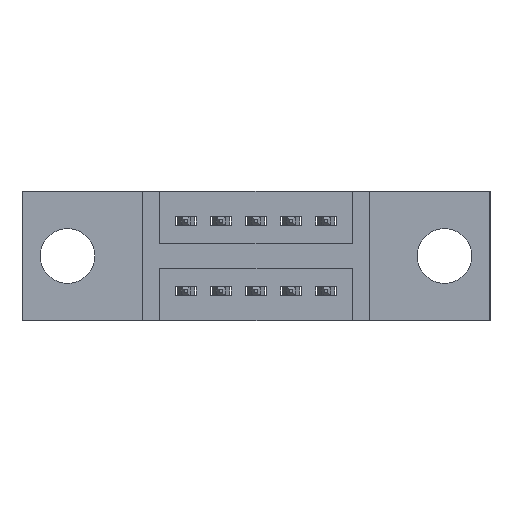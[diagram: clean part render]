
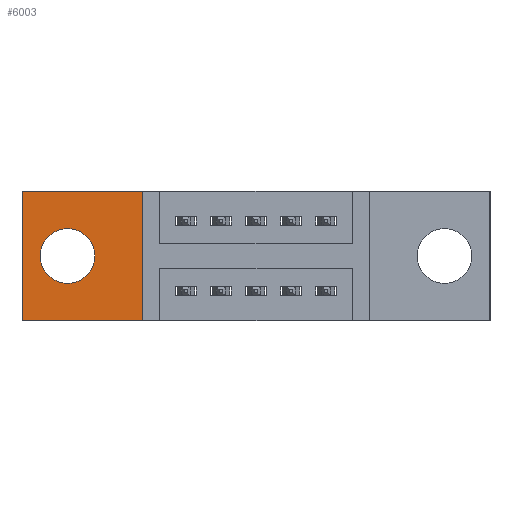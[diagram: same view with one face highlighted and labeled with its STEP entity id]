
A CAD part, front view. The second image highlights one B-rep face of the part: STEP entity #6003.
In plain terms, the highlighted planar face has unit normal (0, -1, 0).
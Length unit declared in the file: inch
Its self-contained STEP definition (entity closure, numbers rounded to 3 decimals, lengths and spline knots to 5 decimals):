
#191 = CIRCLE ( 'NONE', #6354, 0.078 ) ;
#339 = VERTEX_POINT ( 'NONE', #7462 ) ;
#435 = ORIENTED_EDGE ( 'NONE', *, *, #7340, .F. ) ;
#459 = ORIENTED_EDGE ( 'NONE', *, *, #895, .T. ) ;
#604 = CARTESIAN_POINT ( 'NONE',  ( 0.3425, 0.17, 0. ) ) ;
#630 = DIRECTION ( 'NONE',  ( 0., 0., 1. ) ) ;
#660 = DIRECTION ( 'NONE',  ( 1., 0., 0. ) ) ;
#766 = VERTEX_POINT ( 'NONE', #769 ) ;
#769 = CARTESIAN_POINT ( 'NONE',  ( 0.13, 0.17, -0.263 ) ) ;
#827 = ORIENTED_EDGE ( 'NONE', *, *, #8716, .F. ) ;
#895 = EDGE_CURVE ( 'NONE', #339, #7707, #3642, .T. ) ;
#1202 = CARTESIAN_POINT ( 'NONE',  ( 0., 0.17, -0.37 ) ) ;
#1680 = DIRECTION ( 'NONE',  ( 0., 0., -1. ) ) ;
#2078 = VERTEX_POINT ( 'NONE', #5749 ) ;
#2148 = EDGE_CURVE ( 'NONE', #7707, #3746, #3924, .T. ) ;
#2295 = ORIENTED_EDGE ( 'NONE', *, *, #2148, .T. ) ;
#2442 = VECTOR ( 'NONE', #2917, 39.37008 ) ;
#2473 = EDGE_CURVE ( 'NONE', #3746, #4569, #2979, .T. ) ;
#2695 = AXIS2_PLACEMENT_3D ( 'NONE', #4217, #8788, #4899 ) ;
#2917 = DIRECTION ( 'NONE',  ( 0., 0., -1. ) ) ;
#2979 = LINE ( 'NONE', #7596, #4770 ) ;
#3642 = LINE ( 'NONE', #1202, #6885 ) ;
#3746 = VERTEX_POINT ( 'NONE', #5152 ) ;
#3902 = CARTESIAN_POINT ( 'NONE',  ( 0.13, 0.17, -0.185 ) ) ;
#3924 = LINE ( 'NONE', #604, #7162 ) ;
#4132 = FACE_OUTER_BOUND ( 'NONE', #7929, .T. ) ;
#4217 = CARTESIAN_POINT ( 'NONE',  ( 0.13, 0.17, -0.185 ) ) ;
#4569 = VERTEX_POINT ( 'NONE', #7557 ) ;
#4583 = DIRECTION ( 'NONE',  ( 0., 0., -1. ) ) ;
#4770 = VECTOR ( 'NONE', #7552, 39.37008 ) ;
#4899 = DIRECTION ( 'NONE',  ( 0., 0., -1. ) ) ;
#4927 = ORIENTED_EDGE ( 'NONE', *, *, #8807, .T. ) ;
#4945 = CIRCLE ( 'NONE', #2695, 0.078 ) ;
#5152 = CARTESIAN_POINT ( 'NONE',  ( 0.3425, 0.17, 0. ) ) ;
#5584 = CARTESIAN_POINT ( 'NONE',  ( 0.3425, 0.17, -0.37 ) ) ;
#5749 = CARTESIAN_POINT ( 'NONE',  ( 0.13, 0.17, -0.107 ) ) ;
#5813 = DIRECTION ( 'NONE',  ( 0., -1., 0. ) ) ;
#5856 = FACE_BOUND ( 'NONE', #6951, .T. ) ;
#6003 = ADVANCED_FACE ( 'NONE', ( #5856, #4132 ), #7057, .T. ) ;
#6025 = LINE ( 'NONE', #8849, #2442 ) ;
#6354 = AXIS2_PLACEMENT_3D ( 'NONE', #3902, #8492, #4583 ) ;
#6885 = VECTOR ( 'NONE', #660, 39.37008 ) ;
#6951 = EDGE_LOOP ( 'NONE', ( #435, #827 ) ) ;
#7057 = PLANE ( 'NONE',  #7858 ) ;
#7162 = VECTOR ( 'NONE', #630, 39.37008 ) ;
#7340 = EDGE_CURVE ( 'NONE', #2078, #766, #191, .T. ) ;
#7462 = CARTESIAN_POINT ( 'NONE',  ( 0., 0.17, -0.37 ) ) ;
#7552 = DIRECTION ( 'NONE',  ( -1., 0., 0. ) ) ;
#7557 = CARTESIAN_POINT ( 'NONE',  ( 0., 0.17, 0. ) ) ;
#7596 = CARTESIAN_POINT ( 'NONE',  ( 0., 0.17, 0. ) ) ;
#7707 = VERTEX_POINT ( 'NONE', #5584 ) ;
#7725 = CARTESIAN_POINT ( 'NONE',  ( 0., 0.17, -0.37 ) ) ;
#7858 = AXIS2_PLACEMENT_3D ( 'NONE', #7725, #5813, #1680 ) ;
#7929 = EDGE_LOOP ( 'NONE', ( #4927, #459, #2295, #8746 ) ) ;
#8492 = DIRECTION ( 'NONE',  ( 0., -1., 0. ) ) ;
#8716 = EDGE_CURVE ( 'NONE', #766, #2078, #4945, .T. ) ;
#8746 = ORIENTED_EDGE ( 'NONE', *, *, #2473, .T. ) ;
#8788 = DIRECTION ( 'NONE',  ( 0., -1., 0. ) ) ;
#8807 = EDGE_CURVE ( 'NONE', #4569, #339, #6025, .T. ) ;
#8849 = CARTESIAN_POINT ( 'NONE',  ( 0., 0.17, 0. ) ) ;
